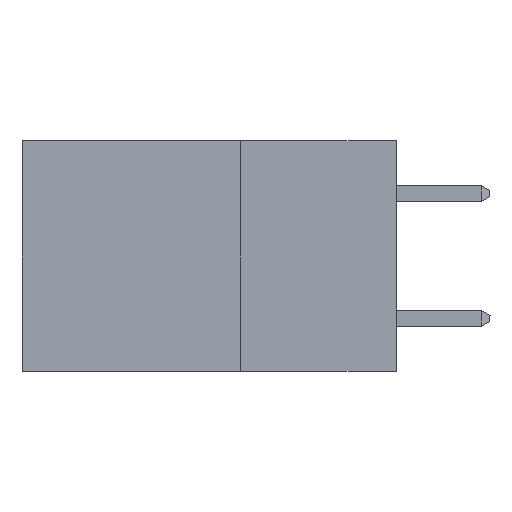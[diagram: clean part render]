
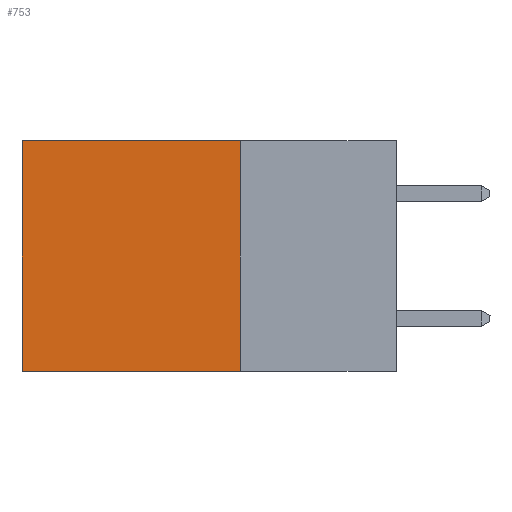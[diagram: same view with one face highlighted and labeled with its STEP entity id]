
A CAD part, left-side view. The second image highlights one B-rep face of the part: STEP entity #753.
In plain terms, the highlighted planar face has unit normal (-1, 0, 0).
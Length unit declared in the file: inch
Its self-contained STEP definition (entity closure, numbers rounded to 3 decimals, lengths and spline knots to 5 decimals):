
#616 = DIRECTION ( 'NONE',  ( 0., 0., -1. ) ) ;
#753 = ADVANCED_FACE ( 'NONE', ( #8526 ), #9978, .F. ) ;
#1157 = CARTESIAN_POINT ( 'NONE',  ( 0.2615, 0.6, 0. ) ) ;
#2040 = ORIENTED_EDGE ( 'NONE', *, *, #9172, .F. ) ;
#2402 = VERTEX_POINT ( 'NONE', #1157 ) ;
#2910 = CARTESIAN_POINT ( 'NONE',  ( 0.2615, 0.25, -0.37 ) ) ;
#2982 = VERTEX_POINT ( 'NONE', #7578 ) ;
#3009 = EDGE_CURVE ( 'NONE', #2982, #2402, #7216, .T. ) ;
#3691 = VECTOR ( 'NONE', #11518, 39.37008 ) ;
#3978 = CARTESIAN_POINT ( 'NONE',  ( 0.2615, 0.25, -0.37 ) ) ;
#6276 = VECTOR ( 'NONE', #7642, 39.37008 ) ;
#6340 = EDGE_CURVE ( 'NONE', #2402, #6976, #8550, .T. ) ;
#6523 = CARTESIAN_POINT ( 'NONE',  ( 0.2615, 0.25, -0.37 ) ) ;
#6594 = DIRECTION ( 'NONE',  ( 0., 0., -1. ) ) ;
#6647 = VECTOR ( 'NONE', #6746, 39.37008 ) ;
#6746 = DIRECTION ( 'NONE',  ( 0., 1., 0. ) ) ;
#6976 = VERTEX_POINT ( 'NONE', #11468 ) ;
#7029 = CARTESIAN_POINT ( 'NONE',  ( 0.2615, 0.6, -0.37 ) ) ;
#7216 = LINE ( 'NONE', #11239, #6647 ) ;
#7474 = EDGE_CURVE ( 'NONE', #11080, #6976, #8659, .T. ) ;
#7548 = ORIENTED_EDGE ( 'NONE', *, *, #7474, .F. ) ;
#7578 = CARTESIAN_POINT ( 'NONE',  ( 0.2615, 0.25, 0. ) ) ;
#7642 = DIRECTION ( 'NONE',  ( 0., 1., 0. ) ) ;
#8526 = FACE_OUTER_BOUND ( 'NONE', #11016, .T. ) ;
#8550 = LINE ( 'NONE', #7029, #3691 ) ;
#8628 = AXIS2_PLACEMENT_3D ( 'NONE', #6523, #9004, #616 ) ;
#8659 = LINE ( 'NONE', #3978, #6276 ) ;
#9004 = DIRECTION ( 'NONE',  ( 1., 0., 0. ) ) ;
#9022 = ORIENTED_EDGE ( 'NONE', *, *, #6340, .T. ) ;
#9171 = LINE ( 'NONE', #2910, #11587 ) ;
#9172 = EDGE_CURVE ( 'NONE', #2982, #11080, #9171, .T. ) ;
#9606 = ORIENTED_EDGE ( 'NONE', *, *, #3009, .T. ) ;
#9978 = PLANE ( 'NONE',  #8628 ) ;
#11016 = EDGE_LOOP ( 'NONE', ( #9022, #7548, #2040, #9606 ) ) ;
#11080 = VERTEX_POINT ( 'NONE', #11104 ) ;
#11104 = CARTESIAN_POINT ( 'NONE',  ( 0.2615, 0.25, -0.37 ) ) ;
#11239 = CARTESIAN_POINT ( 'NONE',  ( 0.2615, 0.25, 0. ) ) ;
#11468 = CARTESIAN_POINT ( 'NONE',  ( 0.2615, 0.6, -0.37 ) ) ;
#11518 = DIRECTION ( 'NONE',  ( 0., 0., -1. ) ) ;
#11587 = VECTOR ( 'NONE', #6594, 39.37008 ) ;
